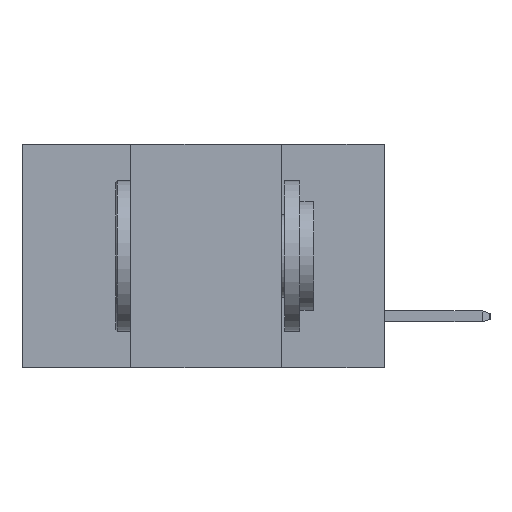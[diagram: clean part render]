
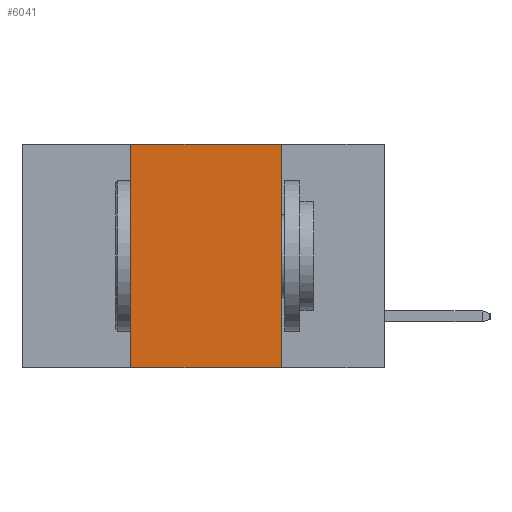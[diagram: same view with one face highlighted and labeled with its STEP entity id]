
A CAD part, left-side view. The second image highlights one B-rep face of the part: STEP entity #6041.
In plain terms, the highlighted planar face has unit normal (-1, 0, 0).
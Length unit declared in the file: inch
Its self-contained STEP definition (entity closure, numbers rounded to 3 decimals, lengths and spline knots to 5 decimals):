
#233 = VECTOR ( 'NONE', #6074, 39.37008 ) ;
#632 = LINE ( 'NONE', #4795, #233 ) ;
#2324 = EDGE_LOOP ( 'NONE', ( #13550, #4260, #4660, #8019 ) ) ;
#2441 = VERTEX_POINT ( 'NONE', #7022 ) ;
#2507 = PLANE ( 'NONE',  #5543 ) ;
#3803 = CARTESIAN_POINT ( 'NONE',  ( 0., 0.17, 0. ) ) ;
#3872 = DIRECTION ( 'NONE',  ( 1., 0., 0. ) ) ;
#3961 = LINE ( 'NONE', #8102, #10685 ) ;
#4260 = ORIENTED_EDGE ( 'NONE', *, *, #14004, .F. ) ;
#4395 = EDGE_CURVE ( 'NONE', #15877, #2441, #11307, .T. ) ;
#4660 = ORIENTED_EDGE ( 'NONE', *, *, #14219, .F. ) ;
#4795 = CARTESIAN_POINT ( 'NONE',  ( 0., 0.42, -0.37 ) ) ;
#5498 = VECTOR ( 'NONE', #13945, 39.37008 ) ;
#5543 = AXIS2_PLACEMENT_3D ( 'NONE', #6382, #3872, #12735 ) ;
#5911 = LINE ( 'NONE', #11433, #5498 ) ;
#6041 = ADVANCED_FACE ( 'NONE', ( #7884 ), #2507, .F. ) ;
#6074 = DIRECTION ( 'NONE',  ( 0., 0., 1. ) ) ;
#6382 = CARTESIAN_POINT ( 'NONE',  ( 0., 0.6, 0. ) ) ;
#7022 = CARTESIAN_POINT ( 'NONE',  ( 0., 0.17, -0.37 ) ) ;
#7080 = CARTESIAN_POINT ( 'NONE',  ( 0., 0.42, -0.37 ) ) ;
#7247 = EDGE_CURVE ( 'NONE', #11779, #2441, #5911, .T. ) ;
#7596 = CARTESIAN_POINT ( 'NONE',  ( 0., 0.42, 0. ) ) ;
#7884 = FACE_OUTER_BOUND ( 'NONE', #2324, .T. ) ;
#8019 = ORIENTED_EDGE ( 'NONE', *, *, #7247, .T. ) ;
#8102 = CARTESIAN_POINT ( 'NONE',  ( 0., 0.6, 0. ) ) ;
#9379 = DIRECTION ( 'NONE',  ( 0., -1., 0. ) ) ;
#10685 = VECTOR ( 'NONE', #9379, 39.37008 ) ;
#10905 = VECTOR ( 'NONE', #12718, 39.37008 ) ;
#11307 = LINE ( 'NONE', #12766, #10905 ) ;
#11370 = VERTEX_POINT ( 'NONE', #7596 ) ;
#11433 = CARTESIAN_POINT ( 'NONE',  ( 0., 0.6, -0.37 ) ) ;
#11779 = VERTEX_POINT ( 'NONE', #7080 ) ;
#12718 = DIRECTION ( 'NONE',  ( 0., 0., -1. ) ) ;
#12735 = DIRECTION ( 'NONE',  ( 0., 0., -1. ) ) ;
#12766 = CARTESIAN_POINT ( 'NONE',  ( 0., 0.17, -0.37 ) ) ;
#13550 = ORIENTED_EDGE ( 'NONE', *, *, #4395, .F. ) ;
#13945 = DIRECTION ( 'NONE',  ( 0., -1., 0. ) ) ;
#14004 = EDGE_CURVE ( 'NONE', #11370, #15877, #3961, .T. ) ;
#14219 = EDGE_CURVE ( 'NONE', #11779, #11370, #632, .T. ) ;
#15877 = VERTEX_POINT ( 'NONE', #3803 ) ;
